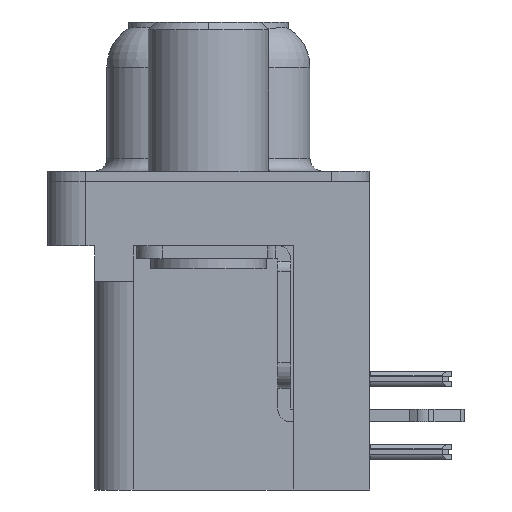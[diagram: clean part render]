
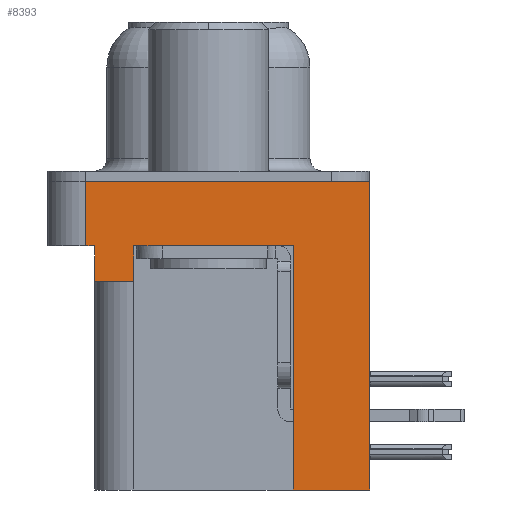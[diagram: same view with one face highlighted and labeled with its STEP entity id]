
A CAD part, left-side view. The second image highlights one B-rep face of the part: STEP entity #8393.
In plain terms, the highlighted planar face has unit normal (-1, 0, 0).
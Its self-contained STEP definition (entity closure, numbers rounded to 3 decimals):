
#1544 = CARTESIAN_POINT ( 'NONE',  ( -3., 4.425, -3.9 ) ) ;
#1708 = ORIENTED_EDGE ( 'NONE', *, *, #27799, .F. ) ;
#1809 = ORIENTED_EDGE ( 'NONE', *, *, #29853, .T. ) ;
#2155 = DIRECTION ( 'NONE',  ( 0., 1., 0. ) ) ;
#2457 = CARTESIAN_POINT ( 'NONE',  ( -3., -6.275, -2.5 ) ) ;
#2955 = DIRECTION ( 'NONE',  ( 0., -1., 0. ) ) ;
#3092 = VERTEX_POINT ( 'NONE', #30189 ) ;
#3172 = FACE_OUTER_BOUND ( 'NONE', #18290, .T. ) ;
#4033 = DIRECTION ( 'NONE',  ( 0., 0., 1. ) ) ;
#4056 = VECTOR ( 'NONE', #2955, 1000. ) ;
#4239 = CARTESIAN_POINT ( 'NONE',  ( -3., 4.775, -2.5 ) ) ;
#4916 = LINE ( 'NONE', #20070, #27941 ) ;
#4961 = CARTESIAN_POINT ( 'NONE',  ( -3., -6.275, -2.5 ) ) ;
#6299 = CARTESIAN_POINT ( 'NONE',  ( -3., -6.275, -12. ) ) ;
#7371 = CARTESIAN_POINT ( 'NONE',  ( -3., -6.275, 0. ) ) ;
#7446 = DIRECTION ( 'NONE',  ( 0., 0., 1. ) ) ;
#7503 = VECTOR ( 'NONE', #4033, 1000. ) ;
#8005 = CARTESIAN_POINT ( 'NONE',  ( -3., -3.295, -12. ) ) ;
#8393 = ADVANCED_FACE ( 'NONE', ( #3172 ), #14708, .T. ) ;
#8916 = VECTOR ( 'NONE', #29050, 1000. ) ;
#9205 = ORIENTED_EDGE ( 'NONE', *, *, #27995, .F. ) ;
#9408 = ORIENTED_EDGE ( 'NONE', *, *, #31468, .T. ) ;
#10447 = VERTEX_POINT ( 'NONE', #26628 ) ;
#11004 = ORIENTED_EDGE ( 'NONE', *, *, #18321, .T. ) ;
#11184 = ORIENTED_EDGE ( 'NONE', *, *, #26826, .F. ) ;
#11379 = VECTOR ( 'NONE', #14863, 1000. ) ;
#12145 = CARTESIAN_POINT ( 'NONE',  ( -3., -3.295, -12. ) ) ;
#12184 = VERTEX_POINT ( 'NONE', #25870 ) ;
#12293 = LINE ( 'NONE', #13231, #18398 ) ;
#12420 = LINE ( 'NONE', #4239, #13923 ) ;
#12926 = ORIENTED_EDGE ( 'NONE', *, *, #22201, .F. ) ;
#13081 = ORIENTED_EDGE ( 'NONE', *, *, #18735, .F. ) ;
#13231 = CARTESIAN_POINT ( 'NONE',  ( -3., 4.425, -3.9 ) ) ;
#13923 = VECTOR ( 'NONE', #29092, 1000. ) ;
#14032 = VERTEX_POINT ( 'NONE', #6299 ) ;
#14465 = CARTESIAN_POINT ( 'NONE',  ( -3., 4.425, -2.5 ) ) ;
#14708 = PLANE ( 'NONE',  #31818 ) ;
#14863 = DIRECTION ( 'NONE',  ( 0., 0., 1. ) ) ;
#14880 = LINE ( 'NONE', #29921, #20283 ) ;
#15021 = DIRECTION ( 'NONE',  ( 0., -1., 0. ) ) ;
#15234 = DIRECTION ( 'NONE',  ( 0., 0., 1. ) ) ;
#15738 = VERTEX_POINT ( 'NONE', #24882 ) ;
#16578 = VECTOR ( 'NONE', #2155, 1000. ) ;
#17051 = CARTESIAN_POINT ( 'NONE',  ( -3., -3.295, -2.5 ) ) ;
#17272 = LINE ( 'NONE', #29243, #28392 ) ;
#17614 = ORIENTED_EDGE ( 'NONE', *, *, #25866, .T. ) ;
#17654 = CARTESIAN_POINT ( 'NONE',  ( -3., -6.275, -2.5 ) ) ;
#17806 = CARTESIAN_POINT ( 'NONE',  ( -3., 2.895, -2.5 ) ) ;
#18290 = EDGE_LOOP ( 'NONE', ( #21656, #9205, #11004, #1708, #13081, #17614, #1809, #11184, #12926, #9408 ) ) ;
#18321 = EDGE_CURVE ( 'NONE', #3092, #24823, #17272, .T. ) ;
#18398 = VECTOR ( 'NONE', #30374, 1000. ) ;
#18735 = EDGE_CURVE ( 'NONE', #12184, #25965, #12293, .T. ) ;
#20070 = CARTESIAN_POINT ( 'NONE',  ( -3., 2.895, -3.9 ) ) ;
#20283 = VECTOR ( 'NONE', #15021, 1000. ) ;
#21656 = ORIENTED_EDGE ( 'NONE', *, *, #25753, .F. ) ;
#22114 = DIRECTION ( 'NONE',  ( -1., 0., 0. ) ) ;
#22201 = EDGE_CURVE ( 'NONE', #14032, #15738, #29634, .T. ) ;
#22557 = VERTEX_POINT ( 'NONE', #7371 ) ;
#22838 = LINE ( 'NONE', #1544, #7503 ) ;
#24044 = CARTESIAN_POINT ( 'NONE',  ( -3., 4.425, -3.9 ) ) ;
#24236 = VERTEX_POINT ( 'NONE', #17051 ) ;
#24823 = VERTEX_POINT ( 'NONE', #14465 ) ;
#24882 = CARTESIAN_POINT ( 'NONE',  ( -3., -3.295, -12. ) ) ;
#25753 = EDGE_CURVE ( 'NONE', #10447, #22557, #14880, .T. ) ;
#25866 = EDGE_CURVE ( 'NONE', #12184, #28473, #4916, .T. ) ;
#25870 = CARTESIAN_POINT ( 'NONE',  ( -3., 2.895, -3.9 ) ) ;
#25965 = VERTEX_POINT ( 'NONE', #24044 ) ;
#26628 = CARTESIAN_POINT ( 'NONE',  ( -3., 4.775, 0. ) ) ;
#26826 = EDGE_CURVE ( 'NONE', #15738, #24236, #29026, .T. ) ;
#26937 = LINE ( 'NONE', #2457, #8916 ) ;
#27799 = EDGE_CURVE ( 'NONE', #25965, #24823, #22838, .T. ) ;
#27941 = VECTOR ( 'NONE', #15234, 1000. ) ;
#27995 = EDGE_CURVE ( 'NONE', #3092, #10447, #12420, .T. ) ;
#28392 = VECTOR ( 'NONE', #29455, 1000. ) ;
#28473 = VERTEX_POINT ( 'NONE', #17806 ) ;
#29026 = LINE ( 'NONE', #8005, #11379 ) ;
#29050 = DIRECTION ( 'NONE',  ( 0., 0., 1. ) ) ;
#29092 = DIRECTION ( 'NONE',  ( 0., 0., 1. ) ) ;
#29243 = CARTESIAN_POINT ( 'NONE',  ( -3., -6.275, -2.5 ) ) ;
#29366 = LINE ( 'NONE', #17654, #4056 ) ;
#29455 = DIRECTION ( 'NONE',  ( 0., -1., 0. ) ) ;
#29634 = LINE ( 'NONE', #12145, #16578 ) ;
#29853 = EDGE_CURVE ( 'NONE', #28473, #24236, #29366, .T. ) ;
#29921 = CARTESIAN_POINT ( 'NONE',  ( -3., -6.275, 0. ) ) ;
#30189 = CARTESIAN_POINT ( 'NONE',  ( -3., 4.775, -2.5 ) ) ;
#30374 = DIRECTION ( 'NONE',  ( 0., 1., 0. ) ) ;
#31468 = EDGE_CURVE ( 'NONE', #14032, #22557, #26937, .T. ) ;
#31818 = AXIS2_PLACEMENT_3D ( 'NONE', #4961, #22114, #7446 ) ;
